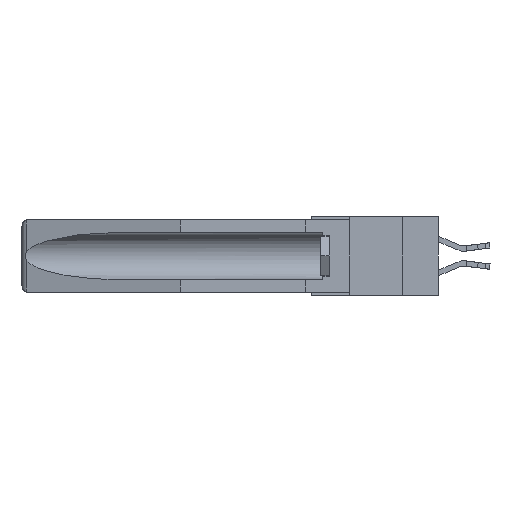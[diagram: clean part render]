
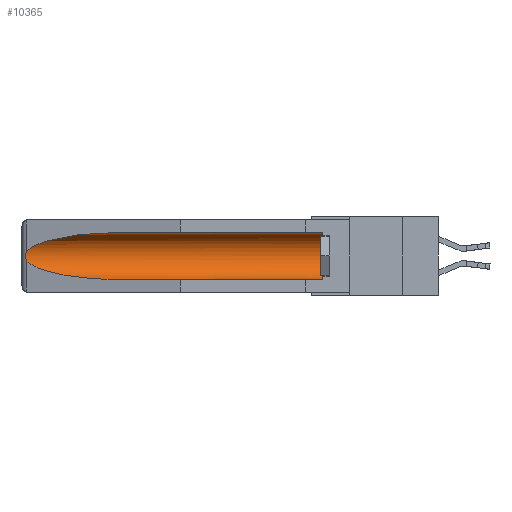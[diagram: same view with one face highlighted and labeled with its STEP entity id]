
A CAD part, left-side view. The second image highlights one B-rep face of the part: STEP entity #10365.
In plain terms, the highlighted cylindrical face has radius 2.857 mm (diameter 5.715 mm), a partial arc.
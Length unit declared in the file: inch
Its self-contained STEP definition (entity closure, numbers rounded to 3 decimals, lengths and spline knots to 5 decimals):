
#197 = VERTEX_POINT ( 'NONE', #7557 ) ;
#427 =( BOUNDED_CURVE ( )  B_SPLINE_CURVE ( 3, ( #7004, #5709, #13981, #11262 ),
 .UNSPECIFIED., .F., .F. ) 
 B_SPLINE_CURVE_WITH_KNOTS ( ( 4, 4 ),
 ( 0.1948, 1.5708 ),
 .UNSPECIFIED. ) 
 CURVE ( )  GEOMETRIC_REPRESENTATION_ITEM ( )  RATIONAL_B_SPLINE_CURVE ( ( 1., 0.848, 0.848, 1. ) ) 
 REPRESENTATION_ITEM ( '' )  );
#508 = CARTESIAN_POINT ( 'NONE',  ( 0.155, -0.30754, -0.284 ) ) ;
#1047 = CARTESIAN_POINT ( 'NONE',  ( 0.26597, 1.52961, -0.15275 ) ) ;
#1790 = CARTESIAN_POINT ( 'NONE',  ( 0.155, 1.07973, -0.284 ) ) ;
#1840 = CARTESIAN_POINT ( 'NONE',  ( 0.155, -0.30754, -0.059 ) ) ;
#2409 = CARTESIAN_POINT ( 'NONE',  ( 0.2673, 1.5327, -0.16383 ) ) ;
#2603 = EDGE_CURVE ( 'NONE', #13961, #8758, #427, .T. ) ;
#2838 = CARTESIAN_POINT ( 'NONE',  ( 0.155, 1.07973, -0.059 ) ) ;
#3276 = LINE ( 'NONE', #508, #16331 ) ;
#3286 = EDGE_CURVE ( 'NONE', #12892, #13961, #6876, .T. ) ;
#3785 = ORIENTED_EDGE ( 'NONE', *, *, #9519, .F. ) ;
#3820 = CARTESIAN_POINT ( 'NONE',  ( 0.26597, 1.5296, -0.19026 ) ) ;
#3836 = LINE ( 'NONE', #1840, #6751 ) ;
#3877 = FACE_OUTER_BOUND ( 'NONE', #7116, .T. ) ;
#3880 = EDGE_CURVE ( 'NONE', #14528, #197, #3836, .T. ) ;
#4596 = CARTESIAN_POINT ( 'NONE',  ( 0.2675, 1.53308, -0.17534 ) ) ;
#5457 = DIRECTION ( 'NONE',  ( 0., 0., 1. ) ) ;
#5709 = CARTESIAN_POINT ( 'NONE',  ( 0.25451, 1.48313, -0.24835 ) ) ;
#6751 = VECTOR ( 'NONE', #7016, 39.37008 ) ;
#6876 = B_SPLINE_CURVE_WITH_KNOTS ( 'NONE', 3,
 ( #15820, #1047, #12732, #2409, #11855, #4596, #7885, #10527, #3820, #15932 ),
 .UNSPECIFIED., .F., .F.,
 ( 4, 2, 2, 2, 4 ),
 ( 0., 0.00029, 0.00058, 0.00087, 0.00117 ),
 .UNSPECIFIED. ) ;
#6881 = CARTESIAN_POINT ( 'NONE',  ( 0.25451, 1.48313, -0.09465 ) ) ;
#6912 = AXIS2_PLACEMENT_3D ( 'NONE', #13662, #14837, #5457 ) ;
#7004 = CARTESIAN_POINT ( 'NONE',  ( 0.26537, 1.52718, -0.19328 ) ) ;
#7016 = DIRECTION ( 'NONE',  ( 0., 1., 0. ) ) ;
#7056 = ORIENTED_EDGE ( 'NONE', *, *, #3880, .T. ) ;
#7116 = EDGE_LOOP ( 'NONE', ( #12470, #10880, #14033, #3785, #14416, #7056 ) ) ;
#7379 = EDGE_CURVE ( 'NONE', #197, #12892, #11114, .T. ) ;
#7557 = CARTESIAN_POINT ( 'NONE',  ( 0.155, 1.07973, -0.059 ) ) ;
#7885 = CARTESIAN_POINT ( 'NONE',  ( 0.2673, 1.53269, -0.17917 ) ) ;
#8758 = VERTEX_POINT ( 'NONE', #1790 ) ;
#8844 = DIRECTION ( 'NONE',  ( 0., 1., 0. ) ) ;
#9519 = EDGE_CURVE ( 'NONE', #11106, #8758, #3276, .T. ) ;
#10365 = ADVANCED_FACE ( 'NONE', ( #3877 ), #12528, .F. ) ;
#10527 = CARTESIAN_POINT ( 'NONE',  ( 0.26655, 1.53094, -0.18657 ) ) ;
#10783 = CIRCLE ( 'NONE', #11929, 0.1125 ) ;
#10880 = ORIENTED_EDGE ( 'NONE', *, *, #3286, .T. ) ;
#11025 = CARTESIAN_POINT ( 'NONE',  ( 0.21114, 1.30732, -0.059 ) ) ;
#11106 = VERTEX_POINT ( 'NONE', #15071 ) ;
#11114 =( BOUNDED_CURVE ( )  B_SPLINE_CURVE ( 3, ( #2838, #11025, #6881, #16133 ),
 .UNSPECIFIED., .F., .T. ) 
 B_SPLINE_CURVE_WITH_KNOTS ( ( 4, 4 ),
 ( 4.71239, 6.08839 ),
 .UNSPECIFIED. ) 
 CURVE ( )  GEOMETRIC_REPRESENTATION_ITEM ( )  RATIONAL_B_SPLINE_CURVE ( ( 1., 0.848, 0.848, 1. ) ) 
 REPRESENTATION_ITEM ( '' )  );
#11262 = CARTESIAN_POINT ( 'NONE',  ( 0.155, 1.07973, -0.284 ) ) ;
#11836 = EDGE_CURVE ( 'NONE', #11106, #14528, #10783, .T. ) ;
#11855 = CARTESIAN_POINT ( 'NONE',  ( 0.2675, 1.53308, -0.16763 ) ) ;
#11929 = AXIS2_PLACEMENT_3D ( 'NONE', #16980, #14116, #15577 ) ;
#12470 = ORIENTED_EDGE ( 'NONE', *, *, #7379, .T. ) ;
#12528 = CYLINDRICAL_SURFACE ( 'NONE', #6912, 0.1125 ) ;
#12732 = CARTESIAN_POINT ( 'NONE',  ( 0.26654, 1.53092, -0.15636 ) ) ;
#12892 = VERTEX_POINT ( 'NONE', #14970 ) ;
#13662 = CARTESIAN_POINT ( 'NONE',  ( 0.155, -0.30754, -0.1715 ) ) ;
#13961 = VERTEX_POINT ( 'NONE', #15738 ) ;
#13981 = CARTESIAN_POINT ( 'NONE',  ( 0.21114, 1.30732, -0.284 ) ) ;
#14033 = ORIENTED_EDGE ( 'NONE', *, *, #2603, .T. ) ;
#14116 = DIRECTION ( 'NONE',  ( 0., -1., 0. ) ) ;
#14416 = ORIENTED_EDGE ( 'NONE', *, *, #11836, .T. ) ;
#14528 = VERTEX_POINT ( 'NONE', #16683 ) ;
#14837 = DIRECTION ( 'NONE',  ( 0., 1., 0. ) ) ;
#14970 = CARTESIAN_POINT ( 'NONE',  ( 0.26537, 1.52718, -0.14972 ) ) ;
#15071 = CARTESIAN_POINT ( 'NONE',  ( 0.155, 0.126, -0.284 ) ) ;
#15577 = DIRECTION ( 'NONE',  ( 0., 0., 1. ) ) ;
#15738 = CARTESIAN_POINT ( 'NONE',  ( 0.26537, 1.52718, -0.19328 ) ) ;
#15820 = CARTESIAN_POINT ( 'NONE',  ( 0.26537, 1.52718, -0.14972 ) ) ;
#15932 = CARTESIAN_POINT ( 'NONE',  ( 0.26537, 1.52718, -0.19328 ) ) ;
#16133 = CARTESIAN_POINT ( 'NONE',  ( 0.26537, 1.52718, -0.14972 ) ) ;
#16331 = VECTOR ( 'NONE', #8844, 39.37008 ) ;
#16683 = CARTESIAN_POINT ( 'NONE',  ( 0.155, 0.126, -0.059 ) ) ;
#16980 = CARTESIAN_POINT ( 'NONE',  ( 0.155, 0.126, -0.1715 ) ) ;
